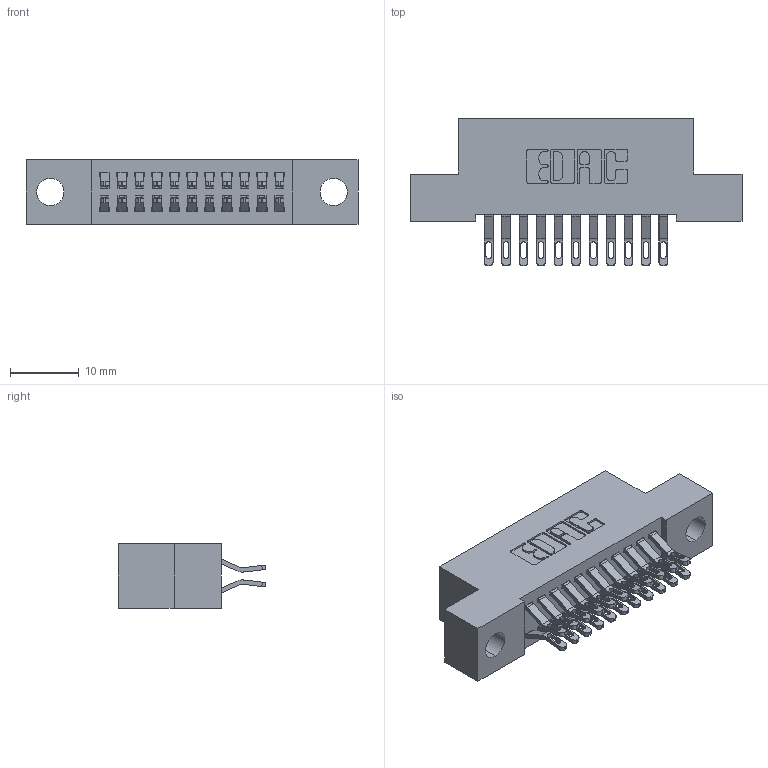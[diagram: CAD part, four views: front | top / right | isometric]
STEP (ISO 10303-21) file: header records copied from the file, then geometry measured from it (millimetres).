
FILE_DESCRIPTION (( 'STEP AP203' ), '1' );
FILE_NAME ('342-022-555-204.STEP', '2018-08-11T00:56:45', ( '' ), ( '' ), 'SwSTEP 2.0', 'SolidWorks 2016', '' );
FILE_SCHEMA (( 'CONFIG_CONTROL_DESIGN' ));
Length unit declared in the file: inch
Products named in the file (3): 342-022-555-204; 342 Part_.156 TH; 345-292-001_555 Tail
Assembly tree (23 placements, depth 2):
  342-022-555-204
    342 Part_.156 TH
    345-292-001_555 Tail  x22
Bounding box: 48.26 x 21.47 x 9.4 mm (x, y, z)
Volume: 4163.5 mm3; surface area: 6050.4 mm2
Topology: 23 solids, 23 shells, 1386 faces, 4325 edges, 2882 vertices
Faces by surface type: plane 814, cylinder 572
Entity records: 11283 total; most frequent: CARTESIAN_POINT 1940, ORIENTED_EDGE 1846, DIRECTION 1683, EDGE_CURVE 923, LINE 775, VECTOR 775, VERTEX_POINT 614, AXIS2_PLACEMENT_3D 454
